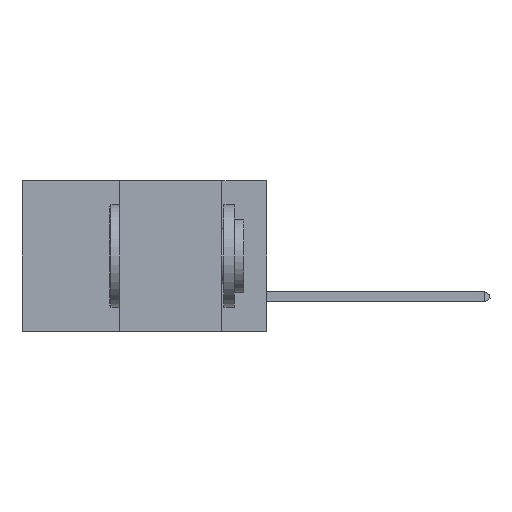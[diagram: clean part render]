
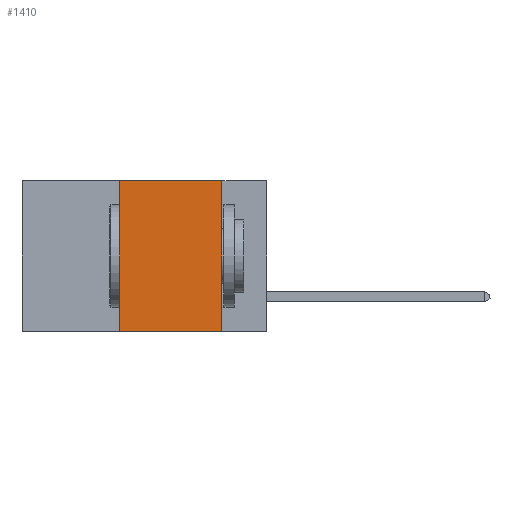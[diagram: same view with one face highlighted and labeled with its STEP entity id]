
A CAD part, left-side view. The second image highlights one B-rep face of the part: STEP entity #1410.
In plain terms, the highlighted planar face has unit normal (-1, 0, 0).
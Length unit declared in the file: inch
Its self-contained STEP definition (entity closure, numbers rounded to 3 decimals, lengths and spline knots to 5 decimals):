
#1184 = VECTOR ( 'NONE', #12495, 39.37008 ) ;
#1410 = ADVANCED_FACE ( 'NONE', ( #8572 ), #10625, .F. ) ;
#1811 = VERTEX_POINT ( 'NONE', #9397 ) ;
#3100 = ORIENTED_EDGE ( 'NONE', *, *, #7317, .F. ) ;
#3120 = VECTOR ( 'NONE', #21904, 39.37008 ) ;
#3468 = EDGE_CURVE ( 'NONE', #20910, #7390, #10826, .T. ) ;
#3509 = AXIS2_PLACEMENT_3D ( 'NONE', #12305, #10296, #10189 ) ;
#3655 = VERTEX_POINT ( 'NONE', #22319 ) ;
#4268 = EDGE_LOOP ( 'NONE', ( #8469, #3100, #4440, #27288 ) ) ;
#4440 = ORIENTED_EDGE ( 'NONE', *, *, #3468, .F. ) ;
#6891 = LINE ( 'NONE', #20948, #1184 ) ;
#7317 = EDGE_CURVE ( 'NONE', #7390, #1811, #19283, .T. ) ;
#7390 = VERTEX_POINT ( 'NONE', #15514 ) ;
#7924 = VECTOR ( 'NONE', #21636, 39.37008 ) ;
#8469 = ORIENTED_EDGE ( 'NONE', *, *, #14921, .F. ) ;
#8572 = FACE_OUTER_BOUND ( 'NONE', #4268, .T. ) ;
#9397 = CARTESIAN_POINT ( 'NONE',  ( 0., 0.11, 0. ) ) ;
#10189 = DIRECTION ( 'NONE',  ( 0., 0., -1. ) ) ;
#10296 = DIRECTION ( 'NONE',  ( 1., 0., 0. ) ) ;
#10625 = PLANE ( 'NONE',  #3509 ) ;
#10826 = LINE ( 'NONE', #25182, #21439 ) ;
#11332 = CARTESIAN_POINT ( 'NONE',  ( 0., 0.6, -0.37 ) ) ;
#12305 = CARTESIAN_POINT ( 'NONE',  ( 0., 0.6, 0. ) ) ;
#12495 = DIRECTION ( 'NONE',  ( 0., 0., -1. ) ) ;
#14921 = EDGE_CURVE ( 'NONE', #1811, #3655, #6891, .T. ) ;
#15514 = CARTESIAN_POINT ( 'NONE',  ( 0., 0.36, 0. ) ) ;
#19283 = LINE ( 'NONE', #19549, #7924 ) ;
#19549 = CARTESIAN_POINT ( 'NONE',  ( 0., 0.6, 0. ) ) ;
#20171 = LINE ( 'NONE', #11332, #3120 ) ;
#20910 = VERTEX_POINT ( 'NONE', #21087 ) ;
#20948 = CARTESIAN_POINT ( 'NONE',  ( 0., 0.11, 0. ) ) ;
#21087 = CARTESIAN_POINT ( 'NONE',  ( 0., 0.36, -0.37 ) ) ;
#21129 = EDGE_CURVE ( 'NONE', #20910, #3655, #20171, .T. ) ;
#21439 = VECTOR ( 'NONE', #25416, 39.37008 ) ;
#21636 = DIRECTION ( 'NONE',  ( 0., -1., 0. ) ) ;
#21904 = DIRECTION ( 'NONE',  ( 0., -1., 0. ) ) ;
#22319 = CARTESIAN_POINT ( 'NONE',  ( 0., 0.11, -0.37 ) ) ;
#25182 = CARTESIAN_POINT ( 'NONE',  ( 0., 0.36, 0. ) ) ;
#25416 = DIRECTION ( 'NONE',  ( 0., 0., 1. ) ) ;
#27288 = ORIENTED_EDGE ( 'NONE', *, *, #21129, .T. ) ;
